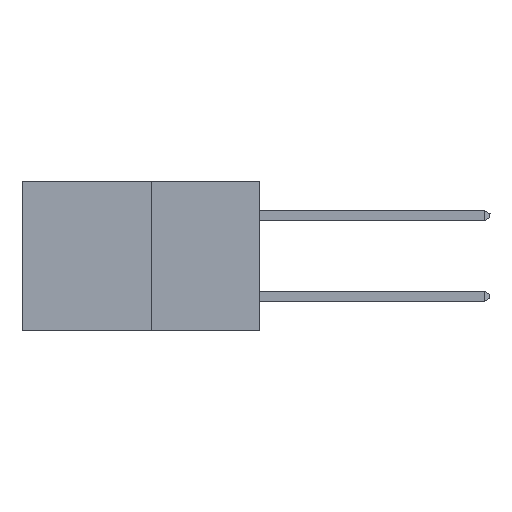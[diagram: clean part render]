
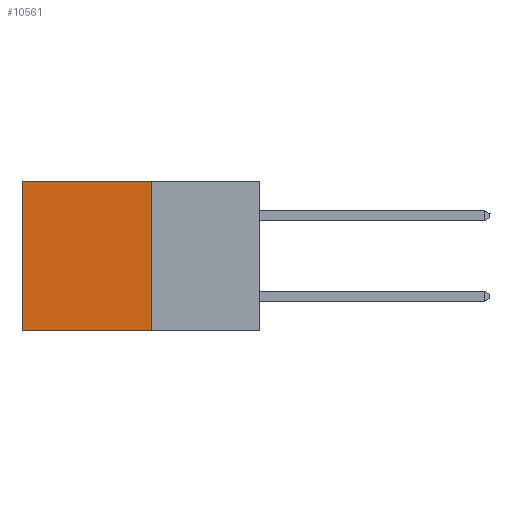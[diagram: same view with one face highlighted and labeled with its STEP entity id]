
A CAD part, left-side view. The second image highlights one B-rep face of the part: STEP entity #10561.
In plain terms, the highlighted planar face has unit normal (-1, 0, 0).
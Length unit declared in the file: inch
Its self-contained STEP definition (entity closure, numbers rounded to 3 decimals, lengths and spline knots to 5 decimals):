
#75 = EDGE_CURVE ( 'NONE', #8473, #3304, #8151, .T. ) ;
#131 = VECTOR ( 'NONE', #293, 39.37008 ) ;
#233 = PLANE ( 'NONE',  #1215 ) ;
#293 = DIRECTION ( 'NONE',  ( 0., 1., 0. ) ) ;
#298 = VERTEX_POINT ( 'NONE', #6961 ) ;
#469 = LINE ( 'NONE', #9086, #131 ) ;
#685 = EDGE_LOOP ( 'NONE', ( #4725, #1044, #1046, #1009 ) ) ;
#728 = CARTESIAN_POINT ( 'NONE',  ( 0.277, 0.27, 0. ) ) ;
#1009 = ORIENTED_EDGE ( 'NONE', *, *, #75, .T. ) ;
#1044 = ORIENTED_EDGE ( 'NONE', *, *, #7591, .F. ) ;
#1046 = ORIENTED_EDGE ( 'NONE', *, *, #2842, .F. ) ;
#1215 = AXIS2_PLACEMENT_3D ( 'NONE', #6078, #4163, #10933 ) ;
#2615 = EDGE_CURVE ( 'NONE', #3304, #5158, #7617, .T. ) ;
#2842 = EDGE_CURVE ( 'NONE', #8473, #298, #3756, .T. ) ;
#2959 = VECTOR ( 'NONE', #12327, 39.37008 ) ;
#3304 = VERTEX_POINT ( 'NONE', #10241 ) ;
#3756 = LINE ( 'NONE', #5230, #6049 ) ;
#4163 = DIRECTION ( 'NONE',  ( 1., 0., 0. ) ) ;
#4641 = CARTESIAN_POINT ( 'NONE',  ( 0.277, 0.59, -0.37 ) ) ;
#4725 = ORIENTED_EDGE ( 'NONE', *, *, #2615, .T. ) ;
#5158 = VERTEX_POINT ( 'NONE', #11297 ) ;
#5230 = CARTESIAN_POINT ( 'NONE',  ( 0.277, 0.27, -0.37 ) ) ;
#5354 = DIRECTION ( 'NONE',  ( 0., 0., -1. ) ) ;
#6049 = VECTOR ( 'NONE', #11560, 39.37008 ) ;
#6078 = CARTESIAN_POINT ( 'NONE',  ( 0.277, 0.27, -0.37 ) ) ;
#6961 = CARTESIAN_POINT ( 'NONE',  ( 0.277, 0.27, -0.37 ) ) ;
#7335 = VECTOR ( 'NONE', #5354, 39.37008 ) ;
#7591 = EDGE_CURVE ( 'NONE', #298, #5158, #469, .T. ) ;
#7617 = LINE ( 'NONE', #4641, #7335 ) ;
#8151 = LINE ( 'NONE', #728, #2959 ) ;
#8473 = VERTEX_POINT ( 'NONE', #10290 ) ;
#9086 = CARTESIAN_POINT ( 'NONE',  ( 0.277, 0.27, -0.37 ) ) ;
#10241 = CARTESIAN_POINT ( 'NONE',  ( 0.277, 0.59, 0. ) ) ;
#10290 = CARTESIAN_POINT ( 'NONE',  ( 0.277, 0.27, 0. ) ) ;
#10561 = ADVANCED_FACE ( 'NONE', ( #10883 ), #233, .F. ) ;
#10883 = FACE_OUTER_BOUND ( 'NONE', #685, .T. ) ;
#10933 = DIRECTION ( 'NONE',  ( 0., 0., -1. ) ) ;
#11297 = CARTESIAN_POINT ( 'NONE',  ( 0.277, 0.59, -0.37 ) ) ;
#11560 = DIRECTION ( 'NONE',  ( 0., 0., -1. ) ) ;
#12327 = DIRECTION ( 'NONE',  ( 0., 1., 0. ) ) ;
